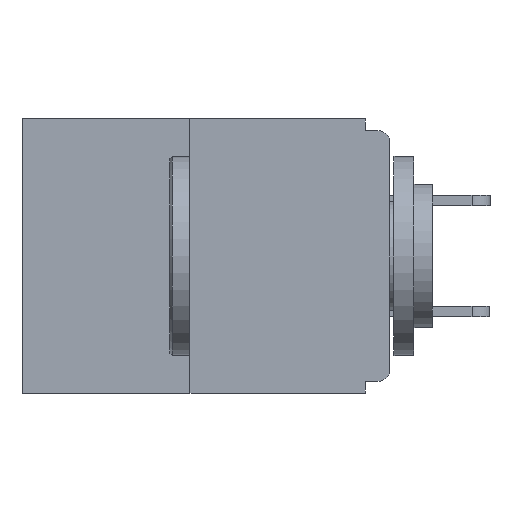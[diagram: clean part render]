
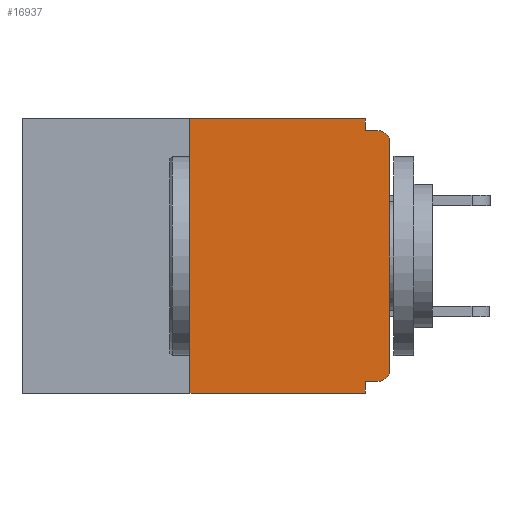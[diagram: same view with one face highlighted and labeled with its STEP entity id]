
A CAD part, left-side view. The second image highlights one B-rep face of the part: STEP entity #16937.
In plain terms, the highlighted planar face has unit normal (-1, 0, 0).
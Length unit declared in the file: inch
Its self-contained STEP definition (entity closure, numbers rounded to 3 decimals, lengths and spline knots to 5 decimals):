
#135 = VERTEX_POINT ( 'NONE', #2605 ) ;
#141 = DIRECTION ( 'NONE',  ( -1., 0., 0. ) ) ;
#155 = CARTESIAN_POINT ( 'NONE',  ( 0., 0., 0. ) ) ;
#209 = DIRECTION ( 'NONE',  ( 0., 0., 1. ) ) ;
#384 = DIRECTION ( 'NONE',  ( -1., 0., 0. ) ) ;
#546 = VERTEX_POINT ( 'NONE', #13329 ) ;
#641 = CARTESIAN_POINT ( 'NONE',  ( 0., 0.015, -0.015 ) ) ;
#1191 = DIRECTION ( 'NONE',  ( 1., 0., 0. ) ) ;
#1234 = VECTOR ( 'NONE', #14316, 39.37008 ) ;
#1474 = CIRCLE ( 'NONE', #4495, 0.015 ) ;
#1773 = ORIENTED_EDGE ( 'NONE', *, *, #18299, .F. ) ;
#2043 = EDGE_CURVE ( 'NONE', #3735, #15548, #6469, .T. ) ;
#2112 = ORIENTED_EDGE ( 'NONE', *, *, #16244, .F. ) ;
#2512 = PLANE ( 'NONE',  #10342 ) ;
#2605 = CARTESIAN_POINT ( 'NONE',  ( 0., 0.031, 0. ) ) ;
#2789 = VECTOR ( 'NONE', #11406, 39.37008 ) ;
#3559 = EDGE_CURVE ( 'NONE', #5263, #8980, #16884, .T. ) ;
#3647 = DIRECTION ( 'NONE',  ( 0., -1., 0. ) ) ;
#3735 = VERTEX_POINT ( 'NONE', #18303 ) ;
#3771 = EDGE_CURVE ( 'NONE', #546, #8980, #1474, .T. ) ;
#3888 = ORIENTED_EDGE ( 'NONE', *, *, #3771, .T. ) ;
#3934 = EDGE_CURVE ( 'NONE', #4271, #135, #10403, .T. ) ;
#4271 = VERTEX_POINT ( 'NONE', #7416 ) ;
#4272 = VERTEX_POINT ( 'NONE', #8884 ) ;
#4495 = AXIS2_PLACEMENT_3D ( 'NONE', #15848, #141, #15912 ) ;
#5059 = EDGE_CURVE ( 'NONE', #4272, #10387, #8091, .T. ) ;
#5263 = VERTEX_POINT ( 'NONE', #12857 ) ;
#5321 = AXIS2_PLACEMENT_3D ( 'NONE', #11507, #384, #12063 ) ;
#5707 = CARTESIAN_POINT ( 'NONE',  ( 0., 0., -0.328 ) ) ;
#6058 = LINE ( 'NONE', #6802, #18173 ) ;
#6098 = LINE ( 'NONE', #10087, #2789 ) ;
#6469 = CIRCLE ( 'NONE', #5321, 0.015 ) ;
#6802 = CARTESIAN_POINT ( 'NONE',  ( 0., 0.25, 0. ) ) ;
#6877 = ORIENTED_EDGE ( 'NONE', *, *, #12607, .F. ) ;
#7416 = CARTESIAN_POINT ( 'NONE',  ( 0., 0.25, 0. ) ) ;
#7420 = ORIENTED_EDGE ( 'NONE', *, *, #18209, .T. ) ;
#7814 = VERTEX_POINT ( 'NONE', #14203 ) ;
#7943 = ORIENTED_EDGE ( 'NONE', *, *, #5059, .T. ) ;
#8091 = LINE ( 'NONE', #16251, #16399 ) ;
#8311 = CARTESIAN_POINT ( 'NONE',  ( 0., 0.46, 0. ) ) ;
#8549 = ORIENTED_EDGE ( 'NONE', *, *, #3559, .F. ) ;
#8857 = CARTESIAN_POINT ( 'NONE',  ( 0., 0., -0.015 ) ) ;
#8884 = CARTESIAN_POINT ( 'NONE',  ( 0., 0.25, -0.343 ) ) ;
#8913 = DIRECTION ( 'NONE',  ( 0., -1., 0. ) ) ;
#8980 = VERTEX_POINT ( 'NONE', #641 ) ;
#9899 = ORIENTED_EDGE ( 'NONE', *, *, #3934, .F. ) ;
#10087 = CARTESIAN_POINT ( 'NONE',  ( 0., 0.031, -0.343 ) ) ;
#10342 = AXIS2_PLACEMENT_3D ( 'NONE', #8311, #1191, #16824 ) ;
#10387 = VERTEX_POINT ( 'NONE', #14099 ) ;
#10403 = LINE ( 'NONE', #15015, #14213 ) ;
#11406 = DIRECTION ( 'NONE',  ( 0., 0., -1. ) ) ;
#11486 = DIRECTION ( 'NONE',  ( 0., 0., 1. ) ) ;
#11507 = CARTESIAN_POINT ( 'NONE',  ( 0., 0.015, -0.313 ) ) ;
#11623 = EDGE_CURVE ( 'NONE', #3735, #7814, #13773, .T. ) ;
#12041 = DIRECTION ( 'NONE',  ( 0., -1., 0. ) ) ;
#12063 = DIRECTION ( 'NONE',  ( 0., 0., -1. ) ) ;
#12607 = EDGE_CURVE ( 'NONE', #7814, #10387, #6098, .T. ) ;
#12857 = CARTESIAN_POINT ( 'NONE',  ( 0., 0.031, -0.015 ) ) ;
#12906 = ORIENTED_EDGE ( 'NONE', *, *, #2043, .T. ) ;
#13232 = DIRECTION ( 'NONE',  ( 0., 0., -1. ) ) ;
#13329 = CARTESIAN_POINT ( 'NONE',  ( 0., 0., -0.03 ) ) ;
#13552 = VECTOR ( 'NONE', #8913, 39.37008 ) ;
#13773 = LINE ( 'NONE', #5707, #1234 ) ;
#14056 = EDGE_LOOP ( 'NONE', ( #9899, #2112, #7943, #6877, #15326, #12906, #7420, #3888, #8549, #1773 ) ) ;
#14086 = LINE ( 'NONE', #155, #15177 ) ;
#14099 = CARTESIAN_POINT ( 'NONE',  ( 0., 0.031, -0.343 ) ) ;
#14203 = CARTESIAN_POINT ( 'NONE',  ( 0., 0.031, -0.328 ) ) ;
#14213 = VECTOR ( 'NONE', #3647, 39.37008 ) ;
#14316 = DIRECTION ( 'NONE',  ( 0., 1., 0. ) ) ;
#14826 = CARTESIAN_POINT ( 'NONE',  ( 0., 0., -0.313 ) ) ;
#14962 = VECTOR ( 'NONE', #13232, 39.37008 ) ;
#15015 = CARTESIAN_POINT ( 'NONE',  ( 0., 0.46, 0. ) ) ;
#15177 = VECTOR ( 'NONE', #209, 39.37008 ) ;
#15326 = ORIENTED_EDGE ( 'NONE', *, *, #11623, .F. ) ;
#15410 = LINE ( 'NONE', #17411, #14962 ) ;
#15548 = VERTEX_POINT ( 'NONE', #14826 ) ;
#15848 = CARTESIAN_POINT ( 'NONE',  ( 0., 0.015, -0.03 ) ) ;
#15912 = DIRECTION ( 'NONE',  ( 0., 0., -1. ) ) ;
#15923 = FACE_OUTER_BOUND ( 'NONE', #14056, .T. ) ;
#16244 = EDGE_CURVE ( 'NONE', #4272, #4271, #6058, .T. ) ;
#16251 = CARTESIAN_POINT ( 'NONE',  ( 0., 0.46, -0.343 ) ) ;
#16399 = VECTOR ( 'NONE', #12041, 39.37008 ) ;
#16824 = DIRECTION ( 'NONE',  ( 0., 0., -1. ) ) ;
#16884 = LINE ( 'NONE', #8857, #13552 ) ;
#16937 = ADVANCED_FACE ( 'NONE', ( #15923 ), #2512, .F. ) ;
#17411 = CARTESIAN_POINT ( 'NONE',  ( 0., 0.031, 0. ) ) ;
#18173 = VECTOR ( 'NONE', #11486, 39.37008 ) ;
#18209 = EDGE_CURVE ( 'NONE', #15548, #546, #14086, .T. ) ;
#18299 = EDGE_CURVE ( 'NONE', #135, #5263, #15410, .T. ) ;
#18303 = CARTESIAN_POINT ( 'NONE',  ( 0., 0.015, -0.328 ) ) ;
